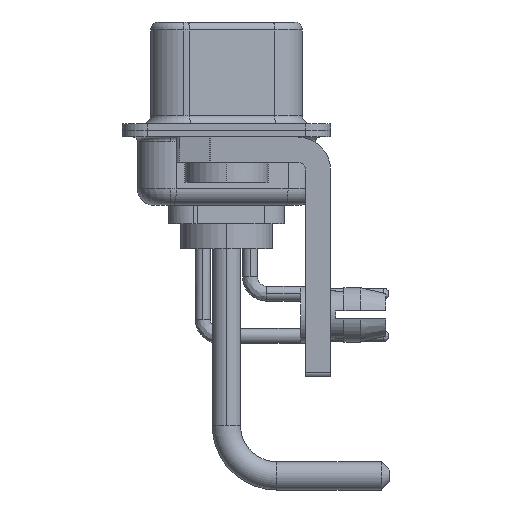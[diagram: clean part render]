
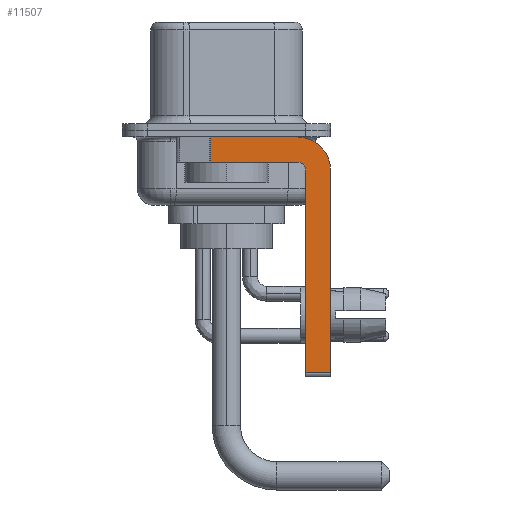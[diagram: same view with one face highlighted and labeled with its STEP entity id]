
A CAD part, left-side view. The second image highlights one B-rep face of the part: STEP entity #11507.
In plain terms, the highlighted planar face has unit normal (-1, 0, 0).
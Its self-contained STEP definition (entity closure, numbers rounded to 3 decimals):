
#1212 = ORIENTED_EDGE ( 'NONE', *, *, #24829, .T. ) ;
#1305 = AXIS2_PLACEMENT_3D ( 'NONE', #19990, #19838, #27570 ) ;
#1400 = ORIENTED_EDGE ( 'NONE', *, *, #13596, .F. ) ;
#2063 = VERTEX_POINT ( 'NONE', #15913 ) ;
#2082 = CARTESIAN_POINT ( 'NONE',  ( -2.9, -4.25, -14.55 ) ) ;
#2084 = DIRECTION ( 'NONE',  ( 0., 0., 1. ) ) ;
#2180 = VERTEX_POINT ( 'NONE', #23637 ) ;
#2233 = CARTESIAN_POINT ( 'NONE',  ( -2.9, -4.25, -0.4 ) ) ;
#2760 = VECTOR ( 'NONE', #11647, 1000. ) ;
#4024 = CARTESIAN_POINT ( 'NONE',  ( -2.9, -6.25, -14.55 ) ) ;
#4111 = EDGE_CURVE ( 'NONE', #21637, #30452, #27855, .T. ) ;
#4264 = CARTESIAN_POINT ( 'NONE',  ( -2.9, 3., -0.4 ) ) ;
#4429 = LINE ( 'NONE', #2082, #2760 ) ;
#5664 = CARTESIAN_POINT ( 'NONE',  ( -2.9, -6.25, -2.4 ) ) ;
#6796 = AXIS2_PLACEMENT_3D ( 'NONE', #19883, #7943, #27133 ) ;
#7943 = DIRECTION ( 'NONE',  ( 1., 0., 0. ) ) ;
#8229 = EDGE_CURVE ( 'NONE', #2180, #2063, #30709, .T. ) ;
#8469 = EDGE_LOOP ( 'NONE', ( #12724, #26426, #1400, #11365, #13439, #1212, #15640, #10090 ) ) ;
#8848 = DIRECTION ( 'NONE',  ( 1., 0., 0. ) ) ;
#9129 = DIRECTION ( 'NONE',  ( 0., -1., 0. ) ) ;
#10090 = ORIENTED_EDGE ( 'NONE', *, *, #12345, .F. ) ;
#10394 = VERTEX_POINT ( 'NONE', #19908 ) ;
#10750 = EDGE_CURVE ( 'NONE', #23157, #12414, #12360, .T. ) ;
#11365 = ORIENTED_EDGE ( 'NONE', *, *, #11393, .F. ) ;
#11393 = EDGE_CURVE ( 'NONE', #2063, #10394, #11853, .T. ) ;
#11507 = ADVANCED_FACE ( 'NONE', ( #23483 ), #20623, .F. ) ;
#11647 = DIRECTION ( 'NONE',  ( 0., -1., 0. ) ) ;
#11853 = CIRCLE ( 'NONE', #1305, 0.5 ) ;
#12345 = EDGE_CURVE ( 'NONE', #30452, #23157, #20330, .T. ) ;
#12360 = LINE ( 'NONE', #29045, #17836 ) ;
#12414 = VERTEX_POINT ( 'NONE', #4024 ) ;
#12724 = ORIENTED_EDGE ( 'NONE', *, *, #4111, .F. ) ;
#13439 = ORIENTED_EDGE ( 'NONE', *, *, #8229, .F. ) ;
#13596 = EDGE_CURVE ( 'NONE', #10394, #14436, #28127, .T. ) ;
#13808 = DIRECTION ( 'NONE',  ( 0., 1., 0. ) ) ;
#13824 = LINE ( 'NONE', #28288, #29819 ) ;
#14436 = VERTEX_POINT ( 'NONE', #27854 ) ;
#15640 = ORIENTED_EDGE ( 'NONE', *, *, #10750, .F. ) ;
#15913 = CARTESIAN_POINT ( 'NONE',  ( -2.9, -4.75, -2.4 ) ) ;
#17836 = VECTOR ( 'NONE', #19574, 1000. ) ;
#18222 = CARTESIAN_POINT ( 'NONE',  ( -2.9, 0.978, -0.4 ) ) ;
#18296 = AXIS2_PLACEMENT_3D ( 'NONE', #28193, #8848, #18425 ) ;
#18425 = DIRECTION ( 'NONE',  ( 0., 0., -1. ) ) ;
#19574 = DIRECTION ( 'NONE',  ( 0., 0., -1. ) ) ;
#19838 = DIRECTION ( 'NONE',  ( -1., 0., 0. ) ) ;
#19883 = CARTESIAN_POINT ( 'NONE',  ( -2.9, -4.25, -2.4 ) ) ;
#19908 = CARTESIAN_POINT ( 'NONE',  ( -2.9, -4.25, -1.9 ) ) ;
#19990 = CARTESIAN_POINT ( 'NONE',  ( -2.9, -4.25, -2.4 ) ) ;
#20330 = CIRCLE ( 'NONE', #6796, 2. ) ;
#20623 = PLANE ( 'NONE',  #18296 ) ;
#21637 = VERTEX_POINT ( 'NONE', #18222 ) ;
#23157 = VERTEX_POINT ( 'NONE', #5664 ) ;
#23237 = VECTOR ( 'NONE', #2084, 1000. ) ;
#23432 = DIRECTION ( 'NONE',  ( 0., 0., -1. ) ) ;
#23483 = FACE_OUTER_BOUND ( 'NONE', #8469, .T. ) ;
#23637 = CARTESIAN_POINT ( 'NONE',  ( -2.9, -4.75, -14.55 ) ) ;
#24829 = EDGE_CURVE ( 'NONE', #2180, #12414, #4429, .T. ) ;
#25275 = EDGE_CURVE ( 'NONE', #21637, #14436, #13824, .T. ) ;
#25759 = CARTESIAN_POINT ( 'NONE',  ( -2.9, -4.25, -1.9 ) ) ;
#26426 = ORIENTED_EDGE ( 'NONE', *, *, #25275, .T. ) ;
#26637 = VECTOR ( 'NONE', #9129, 1000. ) ;
#26946 = VECTOR ( 'NONE', #13808, 1000. ) ;
#27133 = DIRECTION ( 'NONE',  ( 0., 0., -1. ) ) ;
#27570 = DIRECTION ( 'NONE',  ( 0., 0., 1. ) ) ;
#27854 = CARTESIAN_POINT ( 'NONE',  ( -2.9, 0.978, -1.9 ) ) ;
#27855 = LINE ( 'NONE', #4264, #26637 ) ;
#28127 = LINE ( 'NONE', #25759, #26946 ) ;
#28193 = CARTESIAN_POINT ( 'NONE',  ( -2.9, -4.25, -2.4 ) ) ;
#28288 = CARTESIAN_POINT ( 'NONE',  ( -2.9, 0.978, -1.9 ) ) ;
#28326 = CARTESIAN_POINT ( 'NONE',  ( -2.9, -4.75, -14.8 ) ) ;
#29045 = CARTESIAN_POINT ( 'NONE',  ( -2.9, -6.25, -2.4 ) ) ;
#29819 = VECTOR ( 'NONE', #23432, 1000. ) ;
#30452 = VERTEX_POINT ( 'NONE', #2233 ) ;
#30709 = LINE ( 'NONE', #28326, #23237 ) ;
